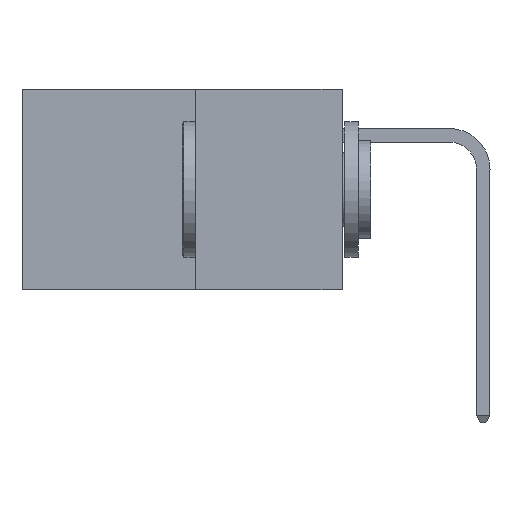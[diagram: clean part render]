
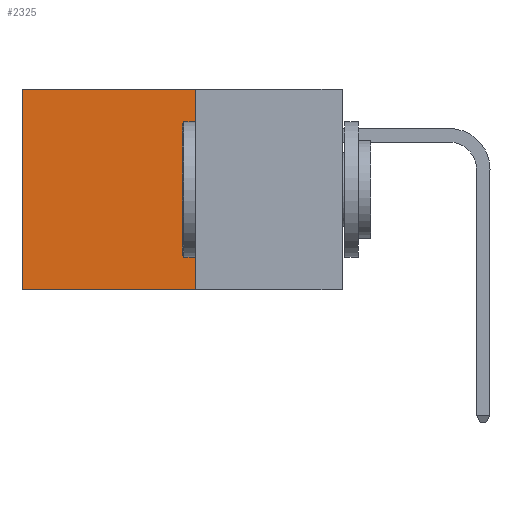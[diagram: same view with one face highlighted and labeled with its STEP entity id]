
A CAD part, left-side view. The second image highlights one B-rep face of the part: STEP entity #2325.
In plain terms, the highlighted planar face has unit normal (-1, 0, 0).
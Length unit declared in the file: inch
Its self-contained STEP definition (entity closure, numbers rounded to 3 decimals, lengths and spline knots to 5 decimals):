
#189 = EDGE_CURVE ( 'NONE', #20797, #8544, #22979, .T. ) ;
#383 = CARTESIAN_POINT ( 'NONE',  ( 0.277, 0.59, -0.37 ) ) ;
#946 = ORIENTED_EDGE ( 'NONE', *, *, #189, .F. ) ;
#2236 = VECTOR ( 'NONE', #22262, 39.37008 ) ;
#2325 = ADVANCED_FACE ( 'NONE', ( #26450 ), #12064, .F. ) ;
#2429 = DIRECTION ( 'NONE',  ( 0., 1., 0. ) ) ;
#2951 = EDGE_CURVE ( 'NONE', #25313, #21402, #23679, .T. ) ;
#3188 = EDGE_LOOP ( 'NONE', ( #17337, #946, #7556, #24908 ) ) ;
#4769 = CARTESIAN_POINT ( 'NONE',  ( 0.277, 0.27, -0.37 ) ) ;
#5898 = AXIS2_PLACEMENT_3D ( 'NONE', #12997, #12970, #19350 ) ;
#6471 = VECTOR ( 'NONE', #18018, 39.37008 ) ;
#7556 = ORIENTED_EDGE ( 'NONE', *, *, #26413, .F. ) ;
#8544 = VERTEX_POINT ( 'NONE', #383 ) ;
#8616 = LINE ( 'NONE', #24288, #2236 ) ;
#8900 = CARTESIAN_POINT ( 'NONE',  ( 0.277, 0.27, 0. ) ) ;
#11021 = CARTESIAN_POINT ( 'NONE',  ( 0.277, 0.59, 0. ) ) ;
#12064 = PLANE ( 'NONE',  #5898 ) ;
#12133 = VECTOR ( 'NONE', #17669, 39.37008 ) ;
#12970 = DIRECTION ( 'NONE',  ( 1., 0., 0. ) ) ;
#12997 = CARTESIAN_POINT ( 'NONE',  ( 0.277, 0.27, -0.37 ) ) ;
#14154 = CARTESIAN_POINT ( 'NONE',  ( 0.277, 0.27, 0. ) ) ;
#17337 = ORIENTED_EDGE ( 'NONE', *, *, #20865, .T. ) ;
#17669 = DIRECTION ( 'NONE',  ( 0., 0., -1. ) ) ;
#17968 = VECTOR ( 'NONE', #2429, 39.37008 ) ;
#18018 = DIRECTION ( 'NONE',  ( 0., 1., 0. ) ) ;
#19350 = DIRECTION ( 'NONE',  ( 0., 0., -1. ) ) ;
#20142 = LINE ( 'NONE', #4769, #12133 ) ;
#20344 = CARTESIAN_POINT ( 'NONE',  ( 0.277, 0.27, -0.37 ) ) ;
#20797 = VERTEX_POINT ( 'NONE', #23743 ) ;
#20865 = EDGE_CURVE ( 'NONE', #21402, #8544, #8616, .T. ) ;
#21402 = VERTEX_POINT ( 'NONE', #11021 ) ;
#22262 = DIRECTION ( 'NONE',  ( 0., 0., -1. ) ) ;
#22979 = LINE ( 'NONE', #20344, #6471 ) ;
#23679 = LINE ( 'NONE', #8900, #17968 ) ;
#23743 = CARTESIAN_POINT ( 'NONE',  ( 0.277, 0.27, -0.37 ) ) ;
#24288 = CARTESIAN_POINT ( 'NONE',  ( 0.277, 0.59, -0.37 ) ) ;
#24908 = ORIENTED_EDGE ( 'NONE', *, *, #2951, .T. ) ;
#25313 = VERTEX_POINT ( 'NONE', #14154 ) ;
#26413 = EDGE_CURVE ( 'NONE', #25313, #20797, #20142, .T. ) ;
#26450 = FACE_OUTER_BOUND ( 'NONE', #3188, .T. ) ;
